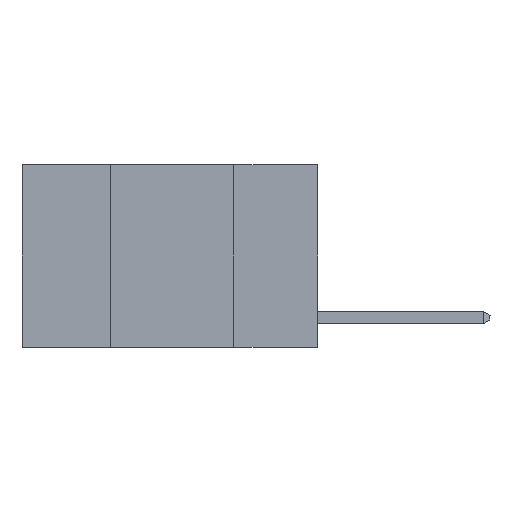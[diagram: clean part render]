
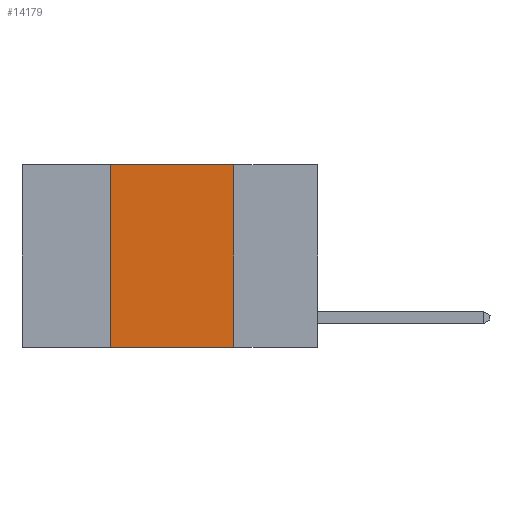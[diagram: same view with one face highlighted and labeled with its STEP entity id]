
A CAD part, left-side view. The second image highlights one B-rep face of the part: STEP entity #14179.
In plain terms, the highlighted planar face has unit normal (-1, 0, 0).
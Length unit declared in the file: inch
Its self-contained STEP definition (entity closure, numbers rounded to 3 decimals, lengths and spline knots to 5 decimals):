
#66 = VERTEX_POINT ( 'NONE', #13903 ) ;
#588 = CARTESIAN_POINT ( 'NONE',  ( 0., 0.42, -0.37 ) ) ;
#868 = EDGE_CURVE ( 'NONE', #14903, #66, #14711, .T. ) ;
#1631 = EDGE_LOOP ( 'NONE', ( #8908, #12559, #2582, #10557 ) ) ;
#2208 = DIRECTION ( 'NONE',  ( 0., 0., -1. ) ) ;
#2556 = LINE ( 'NONE', #17182, #16006 ) ;
#2582 = ORIENTED_EDGE ( 'NONE', *, *, #3811, .F. ) ;
#2755 = AXIS2_PLACEMENT_3D ( 'NONE', #8969, #14318, #2208 ) ;
#3670 = EDGE_CURVE ( 'NONE', #66, #10962, #14894, .T. ) ;
#3811 = EDGE_CURVE ( 'NONE', #17063, #14903, #7028, .T. ) ;
#3844 = VECTOR ( 'NONE', #15889, 39.37008 ) ;
#4191 = CARTESIAN_POINT ( 'NONE',  ( 0., 0.17, 0. ) ) ;
#4997 = VECTOR ( 'NONE', #13225, 39.37008 ) ;
#7028 = LINE ( 'NONE', #12432, #13472 ) ;
#7104 = CARTESIAN_POINT ( 'NONE',  ( 0., 0.17, -0.37 ) ) ;
#7384 = PLANE ( 'NONE',  #2755 ) ;
#8698 = FACE_OUTER_BOUND ( 'NONE', #1631, .T. ) ;
#8908 = ORIENTED_EDGE ( 'NONE', *, *, #3670, .F. ) ;
#8969 = CARTESIAN_POINT ( 'NONE',  ( 0., 0.6, 0. ) ) ;
#10557 = ORIENTED_EDGE ( 'NONE', *, *, #12862, .T. ) ;
#10962 = VERTEX_POINT ( 'NONE', #7104 ) ;
#12432 = CARTESIAN_POINT ( 'NONE',  ( 0., 0.42, 0. ) ) ;
#12559 = ORIENTED_EDGE ( 'NONE', *, *, #868, .F. ) ;
#12697 = DIRECTION ( 'NONE',  ( 0., 0., 1. ) ) ;
#12820 = CARTESIAN_POINT ( 'NONE',  ( 0., 0.42, 0. ) ) ;
#12862 = EDGE_CURVE ( 'NONE', #17063, #10962, #2556, .T. ) ;
#13225 = DIRECTION ( 'NONE',  ( 0., 0., -1. ) ) ;
#13394 = CARTESIAN_POINT ( 'NONE',  ( 0., 0.6, 0. ) ) ;
#13472 = VECTOR ( 'NONE', #12697, 39.37008 ) ;
#13903 = CARTESIAN_POINT ( 'NONE',  ( 0., 0.17, 0. ) ) ;
#14179 = ADVANCED_FACE ( 'NONE', ( #8698 ), #7384, .F. ) ;
#14318 = DIRECTION ( 'NONE',  ( 1., 0., 0. ) ) ;
#14711 = LINE ( 'NONE', #13394, #3844 ) ;
#14894 = LINE ( 'NONE', #4191, #4997 ) ;
#14903 = VERTEX_POINT ( 'NONE', #12820 ) ;
#15889 = DIRECTION ( 'NONE',  ( 0., -1., 0. ) ) ;
#16006 = VECTOR ( 'NONE', #17272, 39.37008 ) ;
#17063 = VERTEX_POINT ( 'NONE', #588 ) ;
#17182 = CARTESIAN_POINT ( 'NONE',  ( 0., 0.6, -0.37 ) ) ;
#17272 = DIRECTION ( 'NONE',  ( 0., -1., 0. ) ) ;
